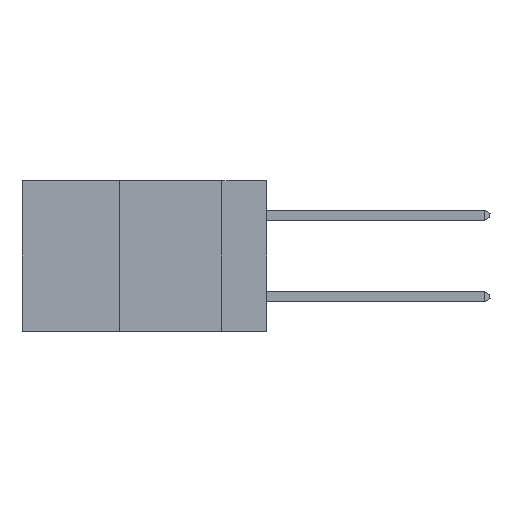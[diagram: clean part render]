
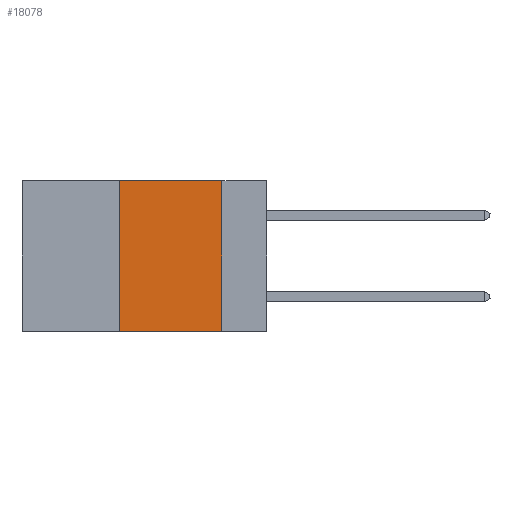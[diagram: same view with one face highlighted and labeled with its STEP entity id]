
A CAD part, left-side view. The second image highlights one B-rep face of the part: STEP entity #18078.
In plain terms, the highlighted planar face has unit normal (-1, 0, 0).
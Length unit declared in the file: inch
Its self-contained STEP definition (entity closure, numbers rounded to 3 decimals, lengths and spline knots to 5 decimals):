
#249 = ORIENTED_EDGE ( 'NONE', *, *, #13875, .F. ) ;
#876 = CARTESIAN_POINT ( 'NONE',  ( 0., 0.6, 0. ) ) ;
#878 = VERTEX_POINT ( 'NONE', #956 ) ;
#956 = CARTESIAN_POINT ( 'NONE',  ( 0., 0.11, -0.37 ) ) ;
#1005 = VECTOR ( 'NONE', #3062, 39.37008 ) ;
#1946 = AXIS2_PLACEMENT_3D ( 'NONE', #16500, #4886, #11916 ) ;
#2136 = VECTOR ( 'NONE', #13323, 39.37008 ) ;
#2184 = CARTESIAN_POINT ( 'NONE',  ( 0., 0.11, 0. ) ) ;
#2297 = VERTEX_POINT ( 'NONE', #4920 ) ;
#3062 = DIRECTION ( 'NONE',  ( 0., -1., 0. ) ) ;
#3225 = CARTESIAN_POINT ( 'NONE',  ( 0., 0.36, 0. ) ) ;
#4336 = VERTEX_POINT ( 'NONE', #14747 ) ;
#4886 = DIRECTION ( 'NONE',  ( 1., 0., 0. ) ) ;
#4920 = CARTESIAN_POINT ( 'NONE',  ( 0., 0.36, 0. ) ) ;
#5752 = LINE ( 'NONE', #14815, #1005 ) ;
#6207 = LINE ( 'NONE', #3225, #2136 ) ;
#7137 = ORIENTED_EDGE ( 'NONE', *, *, #18621, .T. ) ;
#8967 = ORIENTED_EDGE ( 'NONE', *, *, #12206, .F. ) ;
#9865 = ORIENTED_EDGE ( 'NONE', *, *, #10194, .F. ) ;
#10194 = EDGE_CURVE ( 'NONE', #4336, #878, #17570, .T. ) ;
#11010 = VERTEX_POINT ( 'NONE', #12919 ) ;
#11628 = FACE_OUTER_BOUND ( 'NONE', #12315, .T. ) ;
#11916 = DIRECTION ( 'NONE',  ( 0., 0., -1. ) ) ;
#12206 = EDGE_CURVE ( 'NONE', #11010, #2297, #6207, .T. ) ;
#12222 = LINE ( 'NONE', #876, #15644 ) ;
#12315 = EDGE_LOOP ( 'NONE', ( #9865, #249, #8967, #7137 ) ) ;
#12919 = CARTESIAN_POINT ( 'NONE',  ( 0., 0.36, -0.37 ) ) ;
#13323 = DIRECTION ( 'NONE',  ( 0., 0., 1. ) ) ;
#13875 = EDGE_CURVE ( 'NONE', #2297, #4336, #12222, .T. ) ;
#13997 = VECTOR ( 'NONE', #15196, 39.37008 ) ;
#14747 = CARTESIAN_POINT ( 'NONE',  ( 0., 0.11, 0. ) ) ;
#14778 = PLANE ( 'NONE',  #1946 ) ;
#14815 = CARTESIAN_POINT ( 'NONE',  ( 0., 0.6, -0.37 ) ) ;
#15196 = DIRECTION ( 'NONE',  ( 0., 0., -1. ) ) ;
#15644 = VECTOR ( 'NONE', #16937, 39.37008 ) ;
#16500 = CARTESIAN_POINT ( 'NONE',  ( 0., 0.6, 0. ) ) ;
#16937 = DIRECTION ( 'NONE',  ( 0., -1., 0. ) ) ;
#17570 = LINE ( 'NONE', #2184, #13997 ) ;
#18078 = ADVANCED_FACE ( 'NONE', ( #11628 ), #14778, .F. ) ;
#18621 = EDGE_CURVE ( 'NONE', #11010, #878, #5752, .T. ) ;
